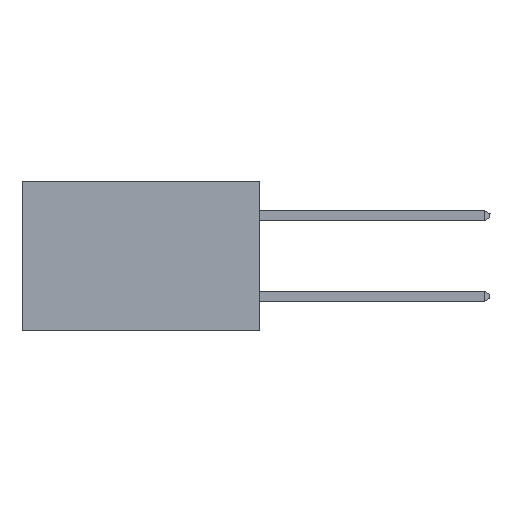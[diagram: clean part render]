
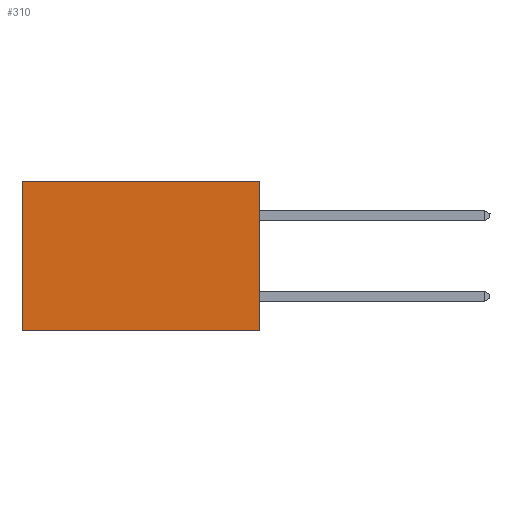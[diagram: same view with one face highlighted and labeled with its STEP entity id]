
A CAD part, left-side view. The second image highlights one B-rep face of the part: STEP entity #310.
In plain terms, the highlighted planar face has unit normal (-1, 0, 0).
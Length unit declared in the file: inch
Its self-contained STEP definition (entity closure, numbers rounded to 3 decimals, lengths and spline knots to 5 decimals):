
#224 = ORIENTED_EDGE ( 'NONE', *, *, #5498, .T. ) ;
#310 = ADVANCED_FACE ( 'NONE', ( #4194 ), #4166, .F. ) ;
#1549 = VERTEX_POINT ( 'NONE', #5481 ) ;
#2395 = VECTOR ( 'NONE', #6460, 39.37008 ) ;
#2945 = EDGE_CURVE ( 'NONE', #9609, #5529, #6014, .T. ) ;
#3266 = CARTESIAN_POINT ( 'NONE',  ( 0.277, 0.59, 0. ) ) ;
#3484 = EDGE_CURVE ( 'NONE', #6052, #1549, #4108, .T. ) ;
#4038 = DIRECTION ( 'NONE',  ( 0., 0., -1. ) ) ;
#4068 = DIRECTION ( 'NONE',  ( 1., 0., 0. ) ) ;
#4108 = LINE ( 'NONE', #6516, #2395 ) ;
#4117 = VECTOR ( 'NONE', #8580, 39.37008 ) ;
#4166 = PLANE ( 'NONE',  #7408 ) ;
#4194 = FACE_OUTER_BOUND ( 'NONE', #5553, .T. ) ;
#4220 = CARTESIAN_POINT ( 'NONE',  ( 0.277, 0., -0.37 ) ) ;
#4572 = CARTESIAN_POINT ( 'NONE',  ( 0.277, 0., 0. ) ) ;
#5139 = DIRECTION ( 'NONE',  ( 0., 1., 0. ) ) ;
#5481 = CARTESIAN_POINT ( 'NONE',  ( 0.277, 0., -0.37 ) ) ;
#5498 = EDGE_CURVE ( 'NONE', #6052, #9609, #8907, .T. ) ;
#5527 = CARTESIAN_POINT ( 'NONE',  ( 0.277, 0., 0. ) ) ;
#5529 = VERTEX_POINT ( 'NONE', #5617 ) ;
#5553 = EDGE_LOOP ( 'NONE', ( #8679, #9034, #9093, #224 ) ) ;
#5617 = CARTESIAN_POINT ( 'NONE',  ( 0.277, 0.59, -0.37 ) ) ;
#5691 = DIRECTION ( 'NONE',  ( 0., 1., 0. ) ) ;
#6014 = LINE ( 'NONE', #8666, #4117 ) ;
#6052 = VERTEX_POINT ( 'NONE', #4572 ) ;
#6430 = CARTESIAN_POINT ( 'NONE',  ( 0.277, 0., -0.37 ) ) ;
#6460 = DIRECTION ( 'NONE',  ( 0., 0., -1. ) ) ;
#6516 = CARTESIAN_POINT ( 'NONE',  ( 0.277, 0., -0.37 ) ) ;
#7408 = AXIS2_PLACEMENT_3D ( 'NONE', #4220, #4068, #4038 ) ;
#8473 = EDGE_CURVE ( 'NONE', #1549, #5529, #9319, .T. ) ;
#8580 = DIRECTION ( 'NONE',  ( 0., 0., -1. ) ) ;
#8666 = CARTESIAN_POINT ( 'NONE',  ( 0.277, 0.59, -0.37 ) ) ;
#8679 = ORIENTED_EDGE ( 'NONE', *, *, #2945, .T. ) ;
#8696 = VECTOR ( 'NONE', #5139, 39.37008 ) ;
#8907 = LINE ( 'NONE', #5527, #8696 ) ;
#9034 = ORIENTED_EDGE ( 'NONE', *, *, #8473, .F. ) ;
#9093 = ORIENTED_EDGE ( 'NONE', *, *, #3484, .F. ) ;
#9111 = VECTOR ( 'NONE', #5691, 39.37008 ) ;
#9319 = LINE ( 'NONE', #6430, #9111 ) ;
#9609 = VERTEX_POINT ( 'NONE', #3266 ) ;
